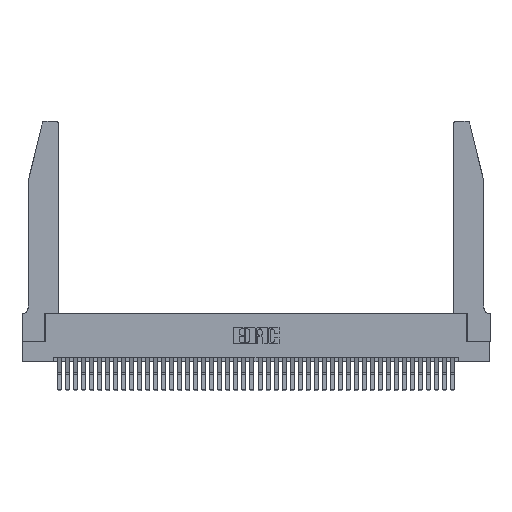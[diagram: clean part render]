
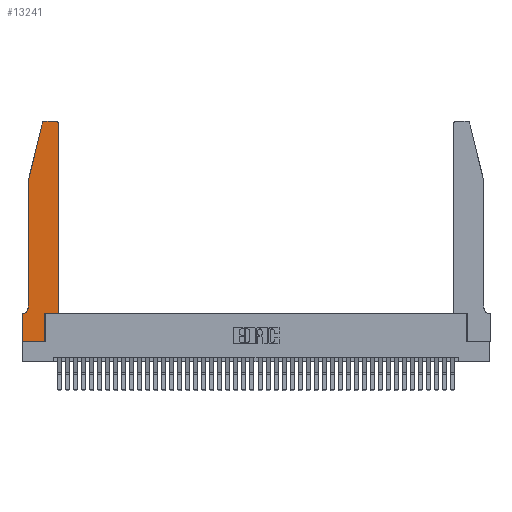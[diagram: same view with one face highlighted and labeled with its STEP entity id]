
A CAD part, top view. The second image highlights one B-rep face of the part: STEP entity #13241.
In plain terms, the highlighted planar face has unit normal (0, 0, 1).
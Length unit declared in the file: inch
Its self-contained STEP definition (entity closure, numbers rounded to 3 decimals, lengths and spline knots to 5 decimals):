
#1215 = LINE ( 'NONE', #16871, #18058 ) ;
#1227 = CARTESIAN_POINT ( 'NONE',  ( 0.0055, 0.42, 0.37 ) ) ;
#1306 = ORIENTED_EDGE ( 'NONE', *, *, #38603, .T. ) ;
#1449 = ORIENTED_EDGE ( 'NONE', *, *, #23009, .T. ) ;
#1586 = CARTESIAN_POINT ( 'NONE',  ( 0.0755, 2., 0.37 ) ) ;
#1677 = DIRECTION ( 'NONE',  ( 1., 0., 0. ) ) ;
#1749 = ORIENTED_EDGE ( 'NONE', *, *, #4128, .T. ) ;
#1789 = VERTEX_POINT ( 'NONE', #27512 ) ;
#1911 = ORIENTED_EDGE ( 'NONE', *, *, #24313, .T. ) ;
#1950 = LINE ( 'NONE', #19563, #9874 ) ;
#2580 = LINE ( 'NONE', #14187, #27186 ) ;
#3167 = VERTEX_POINT ( 'NONE', #24094 ) ;
#3306 = CIRCLE ( 'NONE', #31439, 0.07 ) ;
#3321 = ORIENTED_EDGE ( 'NONE', *, *, #9538, .T. ) ;
#3847 = ORIENTED_EDGE ( 'NONE', *, *, #40473, .T. ) ;
#4112 = VECTOR ( 'NONE', #25037, 39.37008 ) ;
#4128 = EDGE_CURVE ( 'NONE', #31495, #39547, #5517, .T. ) ;
#4203 = EDGE_CURVE ( 'NONE', #39547, #42203, #1215, .T. ) ;
#4594 = CIRCLE ( 'NONE', #9654, 0.03 ) ;
#4690 = DIRECTION ( 'NONE',  ( -1., 0., 0. ) ) ;
#4717 = CARTESIAN_POINT ( 'NONE',  ( 0., 0.35, 0.37 ) ) ;
#5517 = LINE ( 'NONE', #23150, #6555 ) ;
#5714 = CARTESIAN_POINT ( 'NONE',  ( 0.2865, 0.35, 0.37 ) ) ;
#5756 = DIRECTION ( 'NONE',  ( 1., 0., 0. ) ) ;
#6555 = VECTOR ( 'NONE', #36237, 39.37008 ) ;
#7180 = VERTEX_POINT ( 'NONE', #31359 ) ;
#7617 = CARTESIAN_POINT ( 'NONE',  ( 0.284, 2.75, 0.37 ) ) ;
#8283 = ORIENTED_EDGE ( 'NONE', *, *, #25141, .T. ) ;
#8987 = CARTESIAN_POINT ( 'NONE',  ( 0., 0., 0.37 ) ) ;
#9538 = EDGE_CURVE ( 'NONE', #27785, #23967, #2580, .T. ) ;
#9654 = AXIS2_PLACEMENT_3D ( 'NONE', #41412, #21775, #1677 ) ;
#9680 = VECTOR ( 'NONE', #19418, 39.37008 ) ;
#9874 = VECTOR ( 'NONE', #19712, 39.37008 ) ;
#10361 = CARTESIAN_POINT ( 'NONE',  ( 0.0755, 0.42, 0.37 ) ) ;
#10851 = EDGE_CURVE ( 'NONE', #33034, #3167, #24034, .T. ) ;
#11342 = ORIENTED_EDGE ( 'NONE', *, *, #22324, .T. ) ;
#11371 = CARTESIAN_POINT ( 'NONE',  ( 0.4205, 2.72, 0.37 ) ) ;
#12089 = CARTESIAN_POINT ( 'NONE',  ( 0.2865, 0., 0.37 ) ) ;
#12851 = FACE_OUTER_BOUND ( 'NONE', #41118, .T. ) ;
#13241 = ADVANCED_FACE ( 'NONE', ( #12851 ), #18036, .T. ) ;
#14187 = CARTESIAN_POINT ( 'NONE',  ( 0.4505, 0.35, 0.37 ) ) ;
#14728 = DIRECTION ( 'NONE',  ( 1., 0., 0. ) ) ;
#14808 = DIRECTION ( 'NONE',  ( 0., 0., 1. ) ) ;
#15109 = VECTOR ( 'NONE', #42125, 39.37008 ) ;
#15651 = CARTESIAN_POINT ( 'NONE',  ( 0.0755, 2., 0.37 ) ) ;
#15925 = VECTOR ( 'NONE', #5756, 39.37008 ) ;
#16257 = VERTEX_POINT ( 'NONE', #15651 ) ;
#16871 = CARTESIAN_POINT ( 'NONE',  ( 0., 0., 0.37 ) ) ;
#18036 = PLANE ( 'NONE',  #23183 ) ;
#18058 = VECTOR ( 'NONE', #30236, 39.37008 ) ;
#19418 = DIRECTION ( 'NONE',  ( -1., 0., 0. ) ) ;
#19563 = CARTESIAN_POINT ( 'NONE',  ( 0.0755, 2., 0.37 ) ) ;
#19712 = DIRECTION ( 'NONE',  ( 0., -1., 0. ) ) ;
#19814 = LINE ( 'NONE', #1586, #4112 ) ;
#20689 = CARTESIAN_POINT ( 'NONE',  ( 0.0055, 0.35, 0.37 ) ) ;
#21630 = CARTESIAN_POINT ( 'NONE',  ( 0.4505, 0.35, 0.37 ) ) ;
#21775 = DIRECTION ( 'NONE',  ( 0., 0., 1. ) ) ;
#22324 = EDGE_CURVE ( 'NONE', #1789, #16257, #19814, .T. ) ;
#22350 = LINE ( 'NONE', #21630, #38796 ) ;
#22895 = CARTESIAN_POINT ( 'NONE',  ( 0.2605, 2.75, 0.37 ) ) ;
#22969 = EDGE_CURVE ( 'NONE', #3167, #27785, #22350, .T. ) ;
#23009 = EDGE_CURVE ( 'NONE', #35470, #1789, #4594, .T. ) ;
#23024 = ORIENTED_EDGE ( 'NONE', *, *, #4203, .T. ) ;
#23150 = CARTESIAN_POINT ( 'NONE',  ( 0.0755, 0.35, 0.37 ) ) ;
#23183 = AXIS2_PLACEMENT_3D ( 'NONE', #24755, #14808, #37907 ) ;
#23285 = AXIS2_PLACEMENT_3D ( 'NONE', #11371, #34574, #14728 ) ;
#23967 = VERTEX_POINT ( 'NONE', #30239 ) ;
#24034 = LINE ( 'NONE', #5714, #15109 ) ;
#24094 = CARTESIAN_POINT ( 'NONE',  ( 0.2865, 0.35, 0.37 ) ) ;
#24313 = EDGE_CURVE ( 'NONE', #42203, #33034, #25871, .T. ) ;
#24717 = DIRECTION ( 'NONE',  ( 0., 0., -1. ) ) ;
#24755 = CARTESIAN_POINT ( 'NONE',  ( 0., 0.35, 0.37 ) ) ;
#24990 = DIRECTION ( 'NONE',  ( 1., 0., 0. ) ) ;
#25037 = DIRECTION ( 'NONE',  ( -0.239, -0.971, 0. ) ) ;
#25141 = EDGE_CURVE ( 'NONE', #36040, #31495, #3306, .T. ) ;
#25871 = LINE ( 'NONE', #8987, #15925 ) ;
#27186 = VECTOR ( 'NONE', #34034, 39.37008 ) ;
#27407 = LINE ( 'NONE', #22895, #9680 ) ;
#27512 = CARTESIAN_POINT ( 'NONE',  ( 0.25487, 2.72718, 0.37 ) ) ;
#27785 = VERTEX_POINT ( 'NONE', #38891 ) ;
#29810 = ORIENTED_EDGE ( 'NONE', *, *, #31010, .T. ) ;
#30236 = DIRECTION ( 'NONE',  ( 0., -1., 0. ) ) ;
#30239 = CARTESIAN_POINT ( 'NONE',  ( 0.4505, 2.72, 0.37 ) ) ;
#31010 = EDGE_CURVE ( 'NONE', #23967, #7180, #31822, .T. ) ;
#31359 = CARTESIAN_POINT ( 'NONE',  ( 0.4205, 2.75, 0.37 ) ) ;
#31439 = AXIS2_PLACEMENT_3D ( 'NONE', #1227, #24717, #4690 ) ;
#31495 = VERTEX_POINT ( 'NONE', #20689 ) ;
#31822 = CIRCLE ( 'NONE', #23285, 0.03 ) ;
#33034 = VERTEX_POINT ( 'NONE', #12089 ) ;
#33389 = ORIENTED_EDGE ( 'NONE', *, *, #22969, .T. ) ;
#34034 = DIRECTION ( 'NONE',  ( 0., 1., 0. ) ) ;
#34574 = DIRECTION ( 'NONE',  ( 0., 0., 1. ) ) ;
#35470 = VERTEX_POINT ( 'NONE', #7617 ) ;
#36040 = VERTEX_POINT ( 'NONE', #10361 ) ;
#36237 = DIRECTION ( 'NONE',  ( -1., 0., 0. ) ) ;
#37907 = DIRECTION ( 'NONE',  ( 1., 0., 0. ) ) ;
#38603 = EDGE_CURVE ( 'NONE', #16257, #36040, #1950, .T. ) ;
#38796 = VECTOR ( 'NONE', #24990, 39.37008 ) ;
#38891 = CARTESIAN_POINT ( 'NONE',  ( 0.4505, 0.35, 0.37 ) ) ;
#39285 = CARTESIAN_POINT ( 'NONE',  ( 0., 0., 0.37 ) ) ;
#39547 = VERTEX_POINT ( 'NONE', #4717 ) ;
#40069 = ORIENTED_EDGE ( 'NONE', *, *, #10851, .T. ) ;
#40473 = EDGE_CURVE ( 'NONE', #7180, #35470, #27407, .T. ) ;
#41118 = EDGE_LOOP ( 'NONE', ( #3847, #1449, #11342, #1306, #8283, #1749, #23024, #1911, #40069, #33389, #3321, #29810 ) ) ;
#41412 = CARTESIAN_POINT ( 'NONE',  ( 0.284, 2.72, 0.37 ) ) ;
#42125 = DIRECTION ( 'NONE',  ( 0., 1., 0. ) ) ;
#42203 = VERTEX_POINT ( 'NONE', #39285 ) ;
